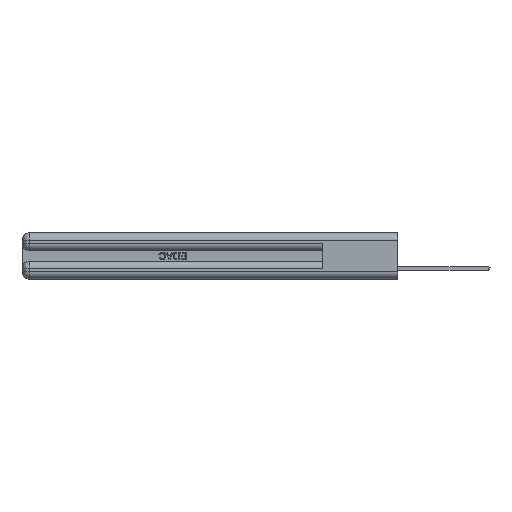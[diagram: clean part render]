
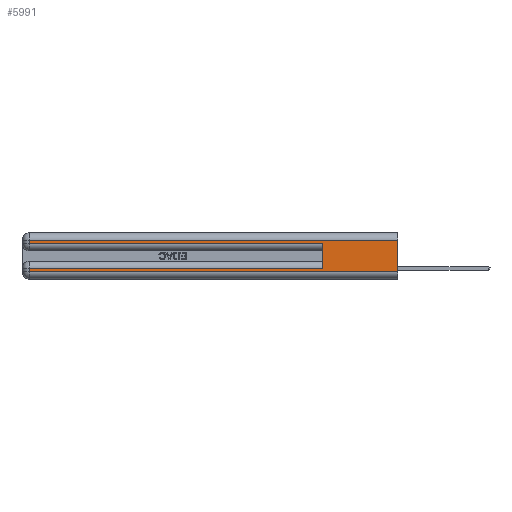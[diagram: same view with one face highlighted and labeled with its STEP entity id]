
A CAD part, left-side view. The second image highlights one B-rep face of the part: STEP entity #5991.
In plain terms, the highlighted planar face has unit normal (-1, 0, 0).
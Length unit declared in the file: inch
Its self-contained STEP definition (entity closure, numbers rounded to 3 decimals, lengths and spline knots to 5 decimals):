
#780 = LINE ( 'NONE', #12634, #33752 ) ;
#2196 = EDGE_CURVE ( 'NONE', #11848, #5029, #780, .T. ) ;
#2422 = EDGE_CURVE ( 'NONE', #9699, #15949, #29852, .T. ) ;
#3790 = EDGE_CURVE ( 'NONE', #9699, #32340, #17183, .T. ) ;
#3813 = ORIENTED_EDGE ( 'NONE', *, *, #21741, .T. ) ;
#4300 = CARTESIAN_POINT ( 'NONE',  ( 0., 2.94, 0.37 ) ) ;
#4431 = ORIENTED_EDGE ( 'NONE', *, *, #38622, .T. ) ;
#5029 = VERTEX_POINT ( 'NONE', #34906 ) ;
#5152 = EDGE_LOOP ( 'NONE', ( #8473, #45208, #34589, #3813, #22217, #22907, #4431, #44160 ) ) ;
#5991 = ADVANCED_FACE ( 'NONE', ( #38307 ), #14479, .F. ) ;
#7351 = LINE ( 'NONE', #36820, #40335 ) ;
#7364 = VERTEX_POINT ( 'NONE', #32257 ) ;
#7747 = VECTOR ( 'NONE', #37723, 39.37008 ) ;
#8400 = CARTESIAN_POINT ( 'NONE',  ( 0., 0.6, 0.285 ) ) ;
#8473 = ORIENTED_EDGE ( 'NONE', *, *, #30257, .F. ) ;
#9699 = VERTEX_POINT ( 'NONE', #34122 ) ;
#9905 = DIRECTION ( 'NONE',  ( 0., 1., 0. ) ) ;
#10616 = CARTESIAN_POINT ( 'NONE',  ( 0., 0., 0.31 ) ) ;
#11045 = DIRECTION ( 'NONE',  ( 0., 0., -1. ) ) ;
#11848 = VERTEX_POINT ( 'NONE', #10616 ) ;
#12005 = CARTESIAN_POINT ( 'NONE',  ( 0., 2.94, 0.06 ) ) ;
#12315 = DIRECTION ( 'NONE',  ( 0., 1., 0. ) ) ;
#12634 = CARTESIAN_POINT ( 'NONE',  ( 0., 0., 0.31 ) ) ;
#14479 = PLANE ( 'NONE',  #27544 ) ;
#14512 = LINE ( 'NONE', #4300, #20628 ) ;
#15949 = VERTEX_POINT ( 'NONE', #28969 ) ;
#16860 = DIRECTION ( 'NONE',  ( 0., 0., -1. ) ) ;
#17006 = CARTESIAN_POINT ( 'NONE',  ( 0., 0., 0.085 ) ) ;
#17183 = LINE ( 'NONE', #17213, #7747 ) ;
#17213 = CARTESIAN_POINT ( 'NONE',  ( 0., 0.6, 0.145 ) ) ;
#18849 = CARTESIAN_POINT ( 'NONE',  ( 0., 0., 0.37 ) ) ;
#19236 = DIRECTION ( 'NONE',  ( 0., -1., 0. ) ) ;
#19305 = DIRECTION ( 'NONE',  ( 1., 0., 0. ) ) ;
#19476 = LINE ( 'NONE', #42629, #21120 ) ;
#20628 = VECTOR ( 'NONE', #11045, 39.37008 ) ;
#21070 = VERTEX_POINT ( 'NONE', #44501 ) ;
#21120 = VECTOR ( 'NONE', #19236, 39.37008 ) ;
#21741 = EDGE_CURVE ( 'NONE', #7364, #32340, #35475, .T. ) ;
#22217 = ORIENTED_EDGE ( 'NONE', *, *, #3790, .F. ) ;
#22720 = CARTESIAN_POINT ( 'NONE',  ( 0., 0., 0.285 ) ) ;
#22907 = ORIENTED_EDGE ( 'NONE', *, *, #2422, .T. ) ;
#23196 = DIRECTION ( 'NONE',  ( 0., -1., 0. ) ) ;
#24169 = EDGE_CURVE ( 'NONE', #39726, #21070, #19476, .T. ) ;
#25247 = DIRECTION ( 'NONE',  ( 0., 0., -1. ) ) ;
#27544 = AXIS2_PLACEMENT_3D ( 'NONE', #18849, #19305, #16860 ) ;
#28969 = CARTESIAN_POINT ( 'NONE',  ( 0., 2.94, 0.085 ) ) ;
#29766 = EDGE_CURVE ( 'NONE', #5029, #7364, #14512, .T. ) ;
#29852 = LINE ( 'NONE', #17006, #32052 ) ;
#30224 = VECTOR ( 'NONE', #25247, 39.37008 ) ;
#30257 = EDGE_CURVE ( 'NONE', #11848, #21070, #7351, .T. ) ;
#32052 = VECTOR ( 'NONE', #9905, 39.37008 ) ;
#32257 = CARTESIAN_POINT ( 'NONE',  ( 0., 2.94, 0.285 ) ) ;
#32340 = VERTEX_POINT ( 'NONE', #8400 ) ;
#33752 = VECTOR ( 'NONE', #12315, 39.37008 ) ;
#34122 = CARTESIAN_POINT ( 'NONE',  ( 0., 0.6, 0.085 ) ) ;
#34589 = ORIENTED_EDGE ( 'NONE', *, *, #29766, .T. ) ;
#34906 = CARTESIAN_POINT ( 'NONE',  ( 0., 2.94, 0.31 ) ) ;
#35475 = LINE ( 'NONE', #22720, #40499 ) ;
#35772 = CARTESIAN_POINT ( 'NONE',  ( 0., 2.94, 0.37 ) ) ;
#36790 = LINE ( 'NONE', #35772, #30224 ) ;
#36820 = CARTESIAN_POINT ( 'NONE',  ( 0., 0., 0.37 ) ) ;
#37723 = DIRECTION ( 'NONE',  ( 0., 0., 1. ) ) ;
#38307 = FACE_OUTER_BOUND ( 'NONE', #5152, .T. ) ;
#38622 = EDGE_CURVE ( 'NONE', #15949, #39726, #36790, .T. ) ;
#39726 = VERTEX_POINT ( 'NONE', #12005 ) ;
#40335 = VECTOR ( 'NONE', #45131, 39.37008 ) ;
#40499 = VECTOR ( 'NONE', #23196, 39.37008 ) ;
#42629 = CARTESIAN_POINT ( 'NONE',  ( 0., 0., 0.06 ) ) ;
#44160 = ORIENTED_EDGE ( 'NONE', *, *, #24169, .T. ) ;
#44501 = CARTESIAN_POINT ( 'NONE',  ( 0., 0., 0.06 ) ) ;
#45131 = DIRECTION ( 'NONE',  ( 0., 0., -1. ) ) ;
#45208 = ORIENTED_EDGE ( 'NONE', *, *, #2196, .T. ) ;
